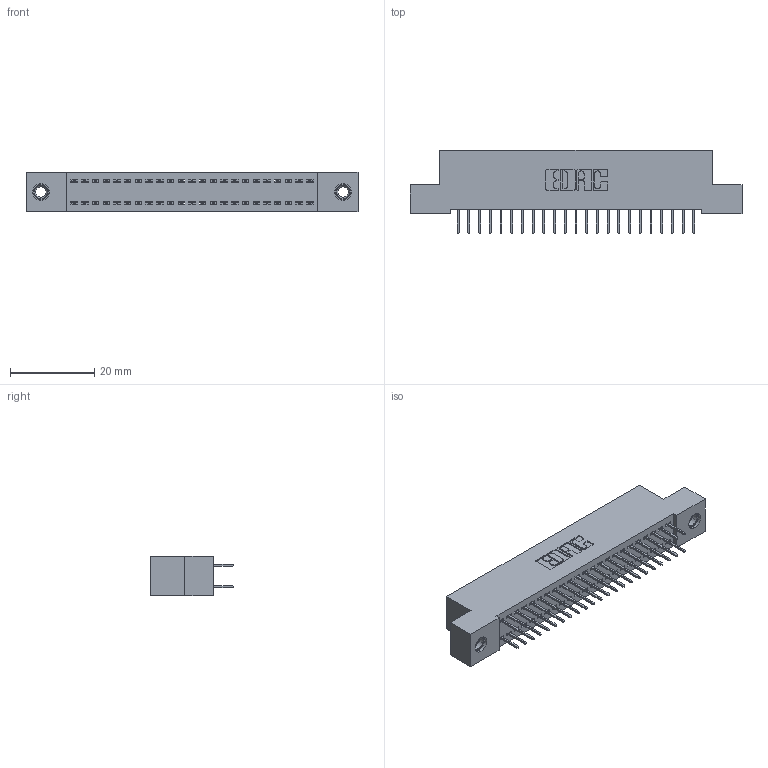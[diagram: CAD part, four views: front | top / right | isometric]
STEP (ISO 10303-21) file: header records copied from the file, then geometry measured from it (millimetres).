
FILE_DESCRIPTION (( 'STEP AP203' ), '1' );
FILE_NAME ('342-046-524-207.STEP', '2019-10-02T20:29:37', ( '' ), ( '' ), 'SwSTEP 2.0', 'SolidWorks 2016', '' );
FILE_SCHEMA (( 'CONFIG_CONTROL_DESIGN' ));
Length unit declared in the file: inch
Products named in the file (4): 342 Part_TI; 345-292-001_345-293-124; 345-250-001_345-250-005-103; 342-046-524-207
Assembly tree (49 placements, depth 2):
  342-046-524-207
    342 Part_TI
    345-292-001_345-293-124  x46
    345-250-001_345-250-005-103  x2
Bounding box: 78.74 x 19.69 x 9.4 mm (x, y, z)
Volume: 6902.5 mm3; surface area: 10612.1 mm2
Topology: 49 solids, 49 shells, 2746 faces, 7749 edges, 4974 vertices
Faces by surface type: plane 2030, cylinder 700, cone 12, torus 4
Entity records: 18382 total; most frequent: CARTESIAN_POINT 3049, ORIENTED_EDGE 2978, DIRECTION 2671, EDGE_CURVE 1489, VECTOR 1345, LINE 1345, VERTEX_POINT 984, AXIS2_PLACEMENT_3D 663
